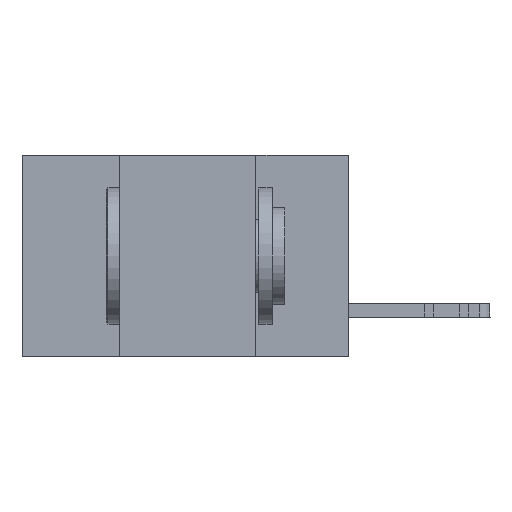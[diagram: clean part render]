
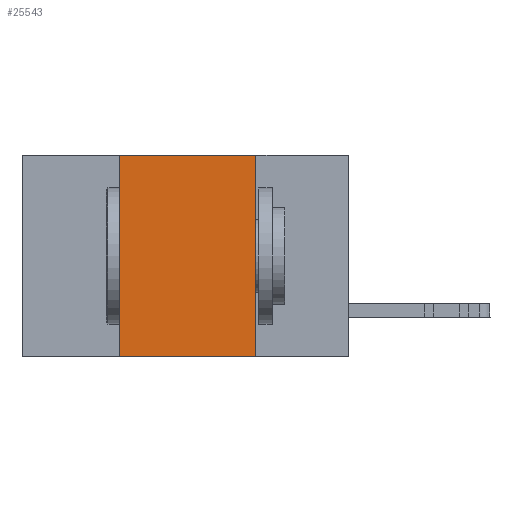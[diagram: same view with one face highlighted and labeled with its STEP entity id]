
A CAD part, left-side view. The second image highlights one B-rep face of the part: STEP entity #25543.
In plain terms, the highlighted planar face has unit normal (-1, 0, 0).
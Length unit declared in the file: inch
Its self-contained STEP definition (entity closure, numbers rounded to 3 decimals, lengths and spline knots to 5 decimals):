
#115 = ORIENTED_EDGE ( 'NONE', *, *, #23873, .F. ) ;
#539 = FACE_OUTER_BOUND ( 'NONE', #2319, .T. ) ;
#2319 = EDGE_LOOP ( 'NONE', ( #27419, #4033, #115, #16874 ) ) ;
#2467 = VERTEX_POINT ( 'NONE', #25607 ) ;
#4033 = ORIENTED_EDGE ( 'NONE', *, *, #30177, .F. ) ;
#4569 = VECTOR ( 'NONE', #19903, 39.37008 ) ;
#5424 = PLANE ( 'NONE',  #26095 ) ;
#5645 = EDGE_CURVE ( 'NONE', #8024, #14805, #17114, .T. ) ;
#5913 = DIRECTION ( 'NONE',  ( 1., 0., 0. ) ) ;
#6708 = CARTESIAN_POINT ( 'NONE',  ( 0., 0.17, -0.37 ) ) ;
#8024 = VERTEX_POINT ( 'NONE', #25645 ) ;
#8777 = VECTOR ( 'NONE', #31742, 39.37008 ) ;
#9009 = VERTEX_POINT ( 'NONE', #17734 ) ;
#9930 = VECTOR ( 'NONE', #29496, 39.37008 ) ;
#10201 = CARTESIAN_POINT ( 'NONE',  ( 0., 0.6, 0. ) ) ;
#10612 = CARTESIAN_POINT ( 'NONE',  ( 0., 0.6, 0. ) ) ;
#12888 = EDGE_CURVE ( 'NONE', #2467, #14805, #15324, .T. ) ;
#14805 = VERTEX_POINT ( 'NONE', #6708 ) ;
#15324 = LINE ( 'NONE', #25140, #9930 ) ;
#15978 = DIRECTION ( 'NONE',  ( 0., 0., -1. ) ) ;
#16874 = ORIENTED_EDGE ( 'NONE', *, *, #12888, .T. ) ;
#17114 = LINE ( 'NONE', #29317, #8777 ) ;
#17734 = CARTESIAN_POINT ( 'NONE',  ( 0., 0.42, 0. ) ) ;
#19903 = DIRECTION ( 'NONE',  ( 0., -1., 0. ) ) ;
#20066 = LINE ( 'NONE', #21876, #22934 ) ;
#21876 = CARTESIAN_POINT ( 'NONE',  ( 0., 0.42, 0. ) ) ;
#22934 = VECTOR ( 'NONE', #27262, 39.37008 ) ;
#23873 = EDGE_CURVE ( 'NONE', #2467, #9009, #20066, .T. ) ;
#25140 = CARTESIAN_POINT ( 'NONE',  ( 0., 0.6, -0.37 ) ) ;
#25543 = ADVANCED_FACE ( 'NONE', ( #539 ), #5424, .F. ) ;
#25607 = CARTESIAN_POINT ( 'NONE',  ( 0., 0.42, -0.37 ) ) ;
#25645 = CARTESIAN_POINT ( 'NONE',  ( 0., 0.17, 0. ) ) ;
#26095 = AXIS2_PLACEMENT_3D ( 'NONE', #10612, #5913, #15978 ) ;
#27262 = DIRECTION ( 'NONE',  ( 0., 0., 1. ) ) ;
#27419 = ORIENTED_EDGE ( 'NONE', *, *, #5645, .F. ) ;
#29317 = CARTESIAN_POINT ( 'NONE',  ( 0., 0.17, 0. ) ) ;
#29496 = DIRECTION ( 'NONE',  ( 0., -1., 0. ) ) ;
#29852 = LINE ( 'NONE', #10201, #4569 ) ;
#30177 = EDGE_CURVE ( 'NONE', #9009, #8024, #29852, .T. ) ;
#31742 = DIRECTION ( 'NONE',  ( 0., 0., -1. ) ) ;
